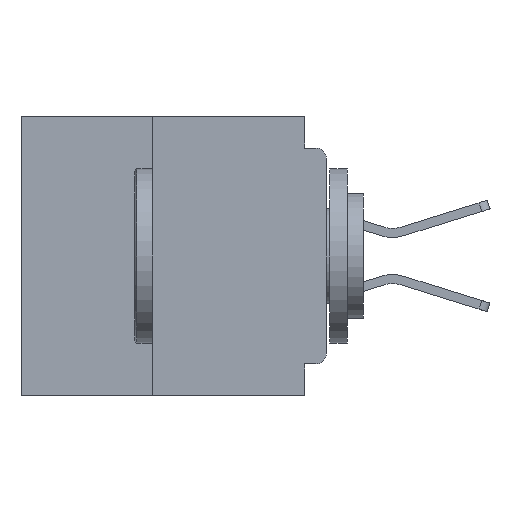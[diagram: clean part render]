
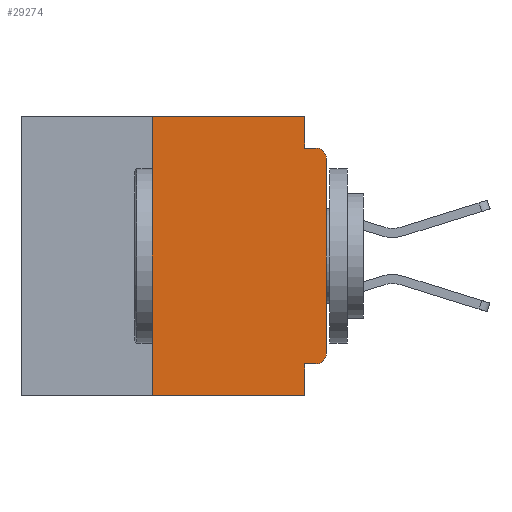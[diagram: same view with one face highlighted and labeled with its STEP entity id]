
A CAD part, left-side view. The second image highlights one B-rep face of the part: STEP entity #29274.
In plain terms, the highlighted planar face has unit normal (-1, 0, 0).
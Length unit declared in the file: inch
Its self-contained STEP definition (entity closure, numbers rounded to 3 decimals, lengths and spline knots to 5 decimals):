
#12 = AXIS2_PLACEMENT_3D ( 'NONE', #9924, #30380, #12938 ) ;
#170 = FACE_OUTER_BOUND ( 'NONE', #36746, .T. ) ;
#874 = VERTEX_POINT ( 'NONE', #8383 ) ;
#1563 = LINE ( 'NONE', #33224, #16658 ) ;
#2390 = VECTOR ( 'NONE', #37412, 39.37008 ) ;
#4688 = VECTOR ( 'NONE', #7534, 39.37008 ) ;
#4930 = VECTOR ( 'NONE', #37992, 39.37008 ) ;
#5348 = EDGE_CURVE ( 'NONE', #36926, #23544, #28212, .T. ) ;
#5903 = VERTEX_POINT ( 'NONE', #35496 ) ;
#6009 = VERTEX_POINT ( 'NONE', #29213 ) ;
#7253 = PLANE ( 'NONE',  #7869 ) ;
#7534 = DIRECTION ( 'NONE',  ( 0., 1., 0. ) ) ;
#7662 = VERTEX_POINT ( 'NONE', #25439 ) ;
#7802 = ORIENTED_EDGE ( 'NONE', *, *, #17734, .F. ) ;
#7869 = AXIS2_PLACEMENT_3D ( 'NONE', #30708, #13263, #33586 ) ;
#8168 = CARTESIAN_POINT ( 'NONE',  ( 0., 0., -0.355 ) ) ;
#8383 = CARTESIAN_POINT ( 'NONE',  ( 0., 0., -0.34 ) ) ;
#8620 = VECTOR ( 'NONE', #11703, 39.37008 ) ;
#9024 = ORIENTED_EDGE ( 'NONE', *, *, #36465, .T. ) ;
#9310 = EDGE_CURVE ( 'NONE', #36926, #874, #19724, .T. ) ;
#9365 = CARTESIAN_POINT ( 'NONE',  ( 0., 0., -0.06 ) ) ;
#9727 = CARTESIAN_POINT ( 'NONE',  ( 0., 0.031, -0.4 ) ) ;
#9924 = CARTESIAN_POINT ( 'NONE',  ( 0., 0.015, -0.34 ) ) ;
#10471 = LINE ( 'NONE', #31718, #2390 ) ;
#10560 = CARTESIAN_POINT ( 'NONE',  ( 0., 0.015, -0.045 ) ) ;
#10731 = VECTOR ( 'NONE', #18628, 39.37008 ) ;
#11227 = AXIS2_PLACEMENT_3D ( 'NONE', #34835, #17504, #37643 ) ;
#11703 = DIRECTION ( 'NONE',  ( 0., -1., 0. ) ) ;
#11825 = EDGE_CURVE ( 'NONE', #6009, #7662, #1563, .T. ) ;
#11896 = LINE ( 'NONE', #22234, #33275 ) ;
#12938 = DIRECTION ( 'NONE',  ( 0., 0., -1. ) ) ;
#13263 = DIRECTION ( 'NONE',  ( 1., 0., 0. ) ) ;
#13661 = ORIENTED_EDGE ( 'NONE', *, *, #5348, .F. ) ;
#13905 = DIRECTION ( 'NONE',  ( 0., -1., 0. ) ) ;
#14339 = ORIENTED_EDGE ( 'NONE', *, *, #17810, .T. ) ;
#14557 = VERTEX_POINT ( 'NONE', #9365 ) ;
#14888 = EDGE_CURVE ( 'NONE', #31364, #31393, #35891, .T. ) ;
#15034 = CIRCLE ( 'NONE', #11227, 0.015 ) ;
#15931 = EDGE_CURVE ( 'NONE', #14557, #31393, #15034, .T. ) ;
#16497 = DIRECTION ( 'NONE',  ( 0., 0., -1. ) ) ;
#16658 = VECTOR ( 'NONE', #18787, 39.37008 ) ;
#17504 = DIRECTION ( 'NONE',  ( -1., 0., 0. ) ) ;
#17734 = EDGE_CURVE ( 'NONE', #7662, #5903, #10471, .T. ) ;
#17810 = EDGE_CURVE ( 'NONE', #6009, #34410, #23346, .T. ) ;
#18574 = LINE ( 'NONE', #9727, #10731 ) ;
#18628 = DIRECTION ( 'NONE',  ( 0., 0., -1. ) ) ;
#18787 = DIRECTION ( 'NONE',  ( 0., 0., 1. ) ) ;
#19241 = ORIENTED_EDGE ( 'NONE', *, *, #34607, .F. ) ;
#19724 = CIRCLE ( 'NONE', #12, 0.015 ) ;
#20110 = ORIENTED_EDGE ( 'NONE', *, *, #32026, .F. ) ;
#22234 = CARTESIAN_POINT ( 'NONE',  ( 0., 0.031, 0. ) ) ;
#23346 = LINE ( 'NONE', #29190, #8620 ) ;
#23544 = VERTEX_POINT ( 'NONE', #25072 ) ;
#25072 = CARTESIAN_POINT ( 'NONE',  ( 0., 0.031, -0.355 ) ) ;
#25439 = CARTESIAN_POINT ( 'NONE',  ( 0., 0.25, 0. ) ) ;
#26539 = CARTESIAN_POINT ( 'NONE',  ( 0., 0., 0. ) ) ;
#27750 = ORIENTED_EDGE ( 'NONE', *, *, #11825, .F. ) ;
#28212 = LINE ( 'NONE', #8168, #4688 ) ;
#28268 = VECTOR ( 'NONE', #13905, 39.37008 ) ;
#28271 = CARTESIAN_POINT ( 'NONE',  ( 0., 0., -0.045 ) ) ;
#28424 = LINE ( 'NONE', #26539, #4930 ) ;
#29190 = CARTESIAN_POINT ( 'NONE',  ( 0., 0.437, -0.4 ) ) ;
#29213 = CARTESIAN_POINT ( 'NONE',  ( 0., 0.25, -0.4 ) ) ;
#29274 = ADVANCED_FACE ( 'NONE', ( #170 ), #7253, .F. ) ;
#29332 = CARTESIAN_POINT ( 'NONE',  ( 0., 0.031, -0.4 ) ) ;
#30380 = DIRECTION ( 'NONE',  ( -1., 0., 0. ) ) ;
#30708 = CARTESIAN_POINT ( 'NONE',  ( 0., 0.437, 0. ) ) ;
#31311 = CARTESIAN_POINT ( 'NONE',  ( 0., 0.015, -0.355 ) ) ;
#31364 = VERTEX_POINT ( 'NONE', #33651 ) ;
#31393 = VERTEX_POINT ( 'NONE', #10560 ) ;
#31718 = CARTESIAN_POINT ( 'NONE',  ( 0., 0.437, 0. ) ) ;
#32026 = EDGE_CURVE ( 'NONE', #5903, #31364, #11896, .T. ) ;
#33224 = CARTESIAN_POINT ( 'NONE',  ( 0., 0.25, -0.4 ) ) ;
#33275 = VECTOR ( 'NONE', #16497, 39.37008 ) ;
#33586 = DIRECTION ( 'NONE',  ( 0., 0., -1. ) ) ;
#33651 = CARTESIAN_POINT ( 'NONE',  ( 0., 0.031, -0.045 ) ) ;
#34114 = ORIENTED_EDGE ( 'NONE', *, *, #15931, .T. ) ;
#34410 = VERTEX_POINT ( 'NONE', #29332 ) ;
#34607 = EDGE_CURVE ( 'NONE', #23544, #34410, #18574, .T. ) ;
#34835 = CARTESIAN_POINT ( 'NONE',  ( 0., 0.015, -0.06 ) ) ;
#35496 = CARTESIAN_POINT ( 'NONE',  ( 0., 0.031, 0. ) ) ;
#35506 = ORIENTED_EDGE ( 'NONE', *, *, #14888, .F. ) ;
#35891 = LINE ( 'NONE', #28271, #28268 ) ;
#36465 = EDGE_CURVE ( 'NONE', #874, #14557, #28424, .T. ) ;
#36746 = EDGE_LOOP ( 'NONE', ( #9024, #34114, #35506, #20110, #7802, #27750, #14339, #19241, #13661, #37109 ) ) ;
#36926 = VERTEX_POINT ( 'NONE', #31311 ) ;
#37109 = ORIENTED_EDGE ( 'NONE', *, *, #9310, .T. ) ;
#37412 = DIRECTION ( 'NONE',  ( 0., -1., 0. ) ) ;
#37643 = DIRECTION ( 'NONE',  ( 0., 0., -1. ) ) ;
#37992 = DIRECTION ( 'NONE',  ( 0., 0., 1. ) ) ;
